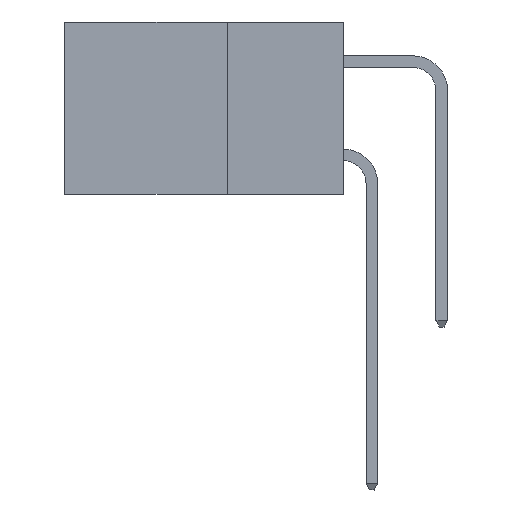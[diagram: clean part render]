
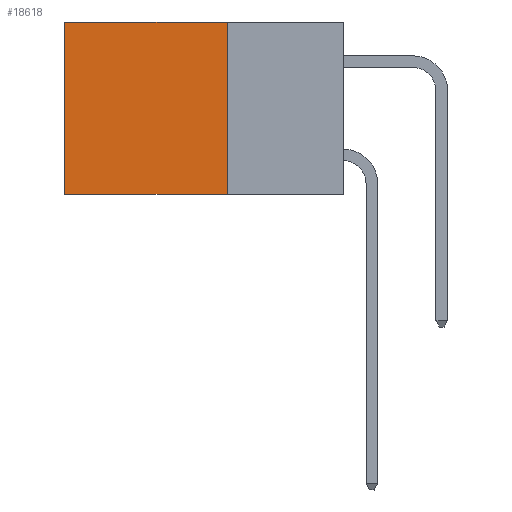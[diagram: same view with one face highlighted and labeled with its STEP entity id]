
A CAD part, left-side view. The second image highlights one B-rep face of the part: STEP entity #18618.
In plain terms, the highlighted planar face has unit normal (-1, 0, 0).
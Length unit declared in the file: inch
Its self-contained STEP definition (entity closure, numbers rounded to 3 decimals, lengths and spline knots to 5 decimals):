
#307 = EDGE_LOOP ( 'NONE', ( #321, #11583, #2403, #23907 ) ) ;
#321 = ORIENTED_EDGE ( 'NONE', *, *, #27444, .T. ) ;
#2247 = EDGE_CURVE ( 'NONE', #11191, #27558, #8746, .T. ) ;
#2308 = CARTESIAN_POINT ( 'NONE',  ( 0.298, 0.25, 0. ) ) ;
#2403 = ORIENTED_EDGE ( 'NONE', *, *, #30086, .F. ) ;
#2683 = AXIS2_PLACEMENT_3D ( 'NONE', #12702, #29140, #15093 ) ;
#4712 = DIRECTION ( 'NONE',  ( 0., 0., -1. ) ) ;
#7277 = LINE ( 'NONE', #17739, #24698 ) ;
#7698 = LINE ( 'NONE', #2308, #19520 ) ;
#8746 = LINE ( 'NONE', #24181, #14269 ) ;
#9350 = CARTESIAN_POINT ( 'NONE',  ( 0.298, 0.25, -0.37 ) ) ;
#9815 = DIRECTION ( 'NONE',  ( 0., 1., 0. ) ) ;
#11191 = VERTEX_POINT ( 'NONE', #19980 ) ;
#11583 = ORIENTED_EDGE ( 'NONE', *, *, #16303, .F. ) ;
#12702 = CARTESIAN_POINT ( 'NONE',  ( 0.298, 0.25, 0. ) ) ;
#14269 = VECTOR ( 'NONE', #9815, 39.37008 ) ;
#14776 = FACE_OUTER_BOUND ( 'NONE', #307, .T. ) ;
#15093 = DIRECTION ( 'NONE',  ( 0., 0., -1. ) ) ;
#16303 = EDGE_CURVE ( 'NONE', #23514, #25564, #18941, .T. ) ;
#16560 = CARTESIAN_POINT ( 'NONE',  ( 0.298, 0.25, -0.37 ) ) ;
#17739 = CARTESIAN_POINT ( 'NONE',  ( 0.298, 0.6, 0. ) ) ;
#18618 = ADVANCED_FACE ( 'NONE', ( #14776 ), #26842, .F. ) ;
#18941 = LINE ( 'NONE', #9350, #25959 ) ;
#19520 = VECTOR ( 'NONE', #4712, 39.37008 ) ;
#19980 = CARTESIAN_POINT ( 'NONE',  ( 0.298, 0.25, 0. ) ) ;
#23514 = VERTEX_POINT ( 'NONE', #16560 ) ;
#23692 = CARTESIAN_POINT ( 'NONE',  ( 0.298, 0.6, 0. ) ) ;
#23907 = ORIENTED_EDGE ( 'NONE', *, *, #2247, .T. ) ;
#24181 = CARTESIAN_POINT ( 'NONE',  ( 0.298, 0.25, 0. ) ) ;
#24698 = VECTOR ( 'NONE', #27219, 39.37008 ) ;
#25564 = VERTEX_POINT ( 'NONE', #29585 ) ;
#25892 = DIRECTION ( 'NONE',  ( 0., 1., 0. ) ) ;
#25959 = VECTOR ( 'NONE', #25892, 39.37008 ) ;
#26842 = PLANE ( 'NONE',  #2683 ) ;
#27219 = DIRECTION ( 'NONE',  ( 0., 0., -1. ) ) ;
#27444 = EDGE_CURVE ( 'NONE', #27558, #25564, #7277, .T. ) ;
#27558 = VERTEX_POINT ( 'NONE', #23692 ) ;
#29140 = DIRECTION ( 'NONE',  ( 1., 0., 0. ) ) ;
#29585 = CARTESIAN_POINT ( 'NONE',  ( 0.298, 0.6, -0.37 ) ) ;
#30086 = EDGE_CURVE ( 'NONE', #11191, #23514, #7698, .T. ) ;
